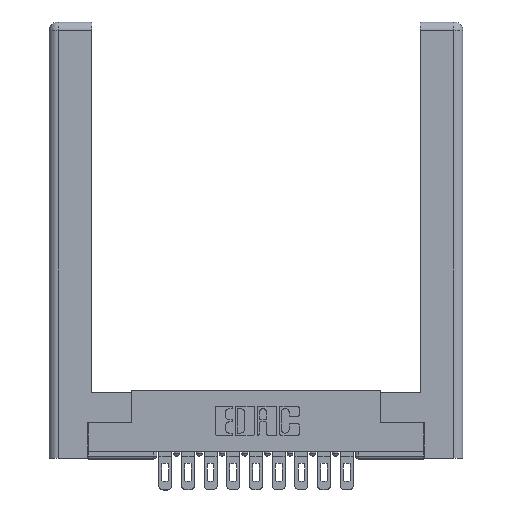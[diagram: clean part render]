
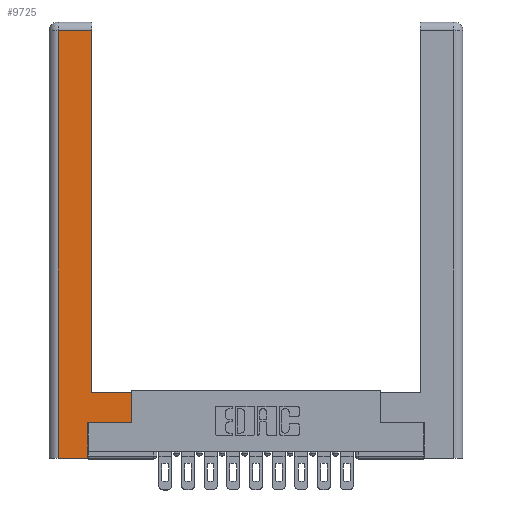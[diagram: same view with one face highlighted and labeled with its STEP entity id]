
A CAD part, top view. The second image highlights one B-rep face of the part: STEP entity #9725.
In plain terms, the highlighted planar face has unit normal (0, 0, 1).
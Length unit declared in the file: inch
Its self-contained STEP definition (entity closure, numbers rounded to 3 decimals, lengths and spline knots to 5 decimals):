
#487 = CARTESIAN_POINT ( 'NONE',  ( 0.0615, 2.94, 0. ) ) ;
#564 = LINE ( 'NONE', #487, #1114 ) ;
#850 = ORIENTED_EDGE ( 'NONE', *, *, #12295, .T. ) ;
#953 = ORIENTED_EDGE ( 'NONE', *, *, #1656, .T. ) ;
#957 = ORIENTED_EDGE ( 'NONE', *, *, #8066, .T. ) ;
#1100 = VERTEX_POINT ( 'NONE', #7253 ) ;
#1114 = VECTOR ( 'NONE', #5015, 39.37008 ) ;
#1339 = DIRECTION ( 'NONE',  ( 0., 0., -1. ) ) ;
#1393 = PLANE ( 'NONE',  #12175 ) ;
#1473 = LINE ( 'NONE', #10968, #13607 ) ;
#1656 = EDGE_CURVE ( 'NONE', #7311, #9506, #10340, .T. ) ;
#1848 = ORIENTED_EDGE ( 'NONE', *, *, #7405, .T. ) ;
#2497 = LINE ( 'NONE', #6456, #14647 ) ;
#2554 = CARTESIAN_POINT ( 'NONE',  ( 0., 0., 0. ) ) ;
#2973 = VECTOR ( 'NONE', #7549, 39.37008 ) ;
#3121 = EDGE_LOOP ( 'NONE', ( #14564, #850, #957, #953, #1848, #12884, #3713, #6019 ) ) ;
#3301 = VERTEX_POINT ( 'NONE', #11423 ) ;
#3435 = EDGE_CURVE ( 'NONE', #9109, #9801, #4992, .T. ) ;
#3713 = ORIENTED_EDGE ( 'NONE', *, *, #3435, .T. ) ;
#3739 = CARTESIAN_POINT ( 'NONE',  ( 0.0615, 0., 0. ) ) ;
#3912 = VECTOR ( 'NONE', #12351, 39.37008 ) ;
#4349 = CARTESIAN_POINT ( 'NONE',  ( 0.265, 0., 0. ) ) ;
#4493 = EDGE_CURVE ( 'NONE', #5567, #5960, #11987, .T. ) ;
#4613 = DIRECTION ( 'NONE',  ( 0., 1., 0. ) ) ;
#4992 = LINE ( 'NONE', #14107, #14067 ) ;
#5015 = DIRECTION ( 'NONE',  ( -1., 0., 0. ) ) ;
#5567 = VERTEX_POINT ( 'NONE', #13019 ) ;
#5960 = VERTEX_POINT ( 'NONE', #13094 ) ;
#6019 = ORIENTED_EDGE ( 'NONE', *, *, #14920, .T. ) ;
#6080 = CARTESIAN_POINT ( 'NONE',  ( 0.565, 0.245, 0. ) ) ;
#6351 = CARTESIAN_POINT ( 'NONE',  ( 0.565, 0.245, 0. ) ) ;
#6456 = CARTESIAN_POINT ( 'NONE',  ( 0.295, 0.45, 0. ) ) ;
#7253 = CARTESIAN_POINT ( 'NONE',  ( 0.265, 0.245, 0. ) ) ;
#7311 = VERTEX_POINT ( 'NONE', #3739 ) ;
#7330 = DIRECTION ( 'NONE',  ( 0., 1., 0. ) ) ;
#7405 = EDGE_CURVE ( 'NONE', #9506, #1100, #13794, .T. ) ;
#7549 = DIRECTION ( 'NONE',  ( 1., 0., 0. ) ) ;
#8066 = EDGE_CURVE ( 'NONE', #3301, #7311, #1473, .T. ) ;
#8740 = FACE_OUTER_BOUND ( 'NONE', #3121, .T. ) ;
#8805 = DIRECTION ( 'NONE',  ( 0., -1., 0. ) ) ;
#8833 = DIRECTION ( 'NONE',  ( -1., 0., 0. ) ) ;
#8848 = VECTOR ( 'NONE', #13304, 39.37008 ) ;
#9109 = VERTEX_POINT ( 'NONE', #6080 ) ;
#9506 = VERTEX_POINT ( 'NONE', #4349 ) ;
#9725 = ADVANCED_FACE ( 'NONE', ( #8740 ), #1393, .F. ) ;
#9801 = VERTEX_POINT ( 'NONE', #13140 ) ;
#10340 = LINE ( 'NONE', #12408, #2973 ) ;
#10623 = EDGE_CURVE ( 'NONE', #1100, #9109, #15177, .T. ) ;
#10968 = CARTESIAN_POINT ( 'NONE',  ( 0.0615, 0., 0. ) ) ;
#11423 = CARTESIAN_POINT ( 'NONE',  ( 0.0615, 2.94, 0. ) ) ;
#11957 = DIRECTION ( 'NONE',  ( -1., 0., 0. ) ) ;
#11987 = LINE ( 'NONE', #13399, #8848 ) ;
#12114 = VECTOR ( 'NONE', #7330, 39.37008 ) ;
#12175 = AXIS2_PLACEMENT_3D ( 'NONE', #2554, #1339, #11957 ) ;
#12295 = EDGE_CURVE ( 'NONE', #5960, #3301, #564, .T. ) ;
#12351 = DIRECTION ( 'NONE',  ( 1., 0., 0. ) ) ;
#12408 = CARTESIAN_POINT ( 'NONE',  ( 0.265, 0., 0. ) ) ;
#12884 = ORIENTED_EDGE ( 'NONE', *, *, #10623, .T. ) ;
#13019 = CARTESIAN_POINT ( 'NONE',  ( 0.295, 0.45, 0. ) ) ;
#13094 = CARTESIAN_POINT ( 'NONE',  ( 0.295, 2.94, 0. ) ) ;
#13140 = CARTESIAN_POINT ( 'NONE',  ( 0.565, 0.45, 0. ) ) ;
#13210 = CARTESIAN_POINT ( 'NONE',  ( 0.265, 0.245, 0. ) ) ;
#13304 = DIRECTION ( 'NONE',  ( 0., 1., 0. ) ) ;
#13399 = CARTESIAN_POINT ( 'NONE',  ( 0.295, 3., 0. ) ) ;
#13607 = VECTOR ( 'NONE', #8805, 39.37008 ) ;
#13794 = LINE ( 'NONE', #13210, #12114 ) ;
#14067 = VECTOR ( 'NONE', #4613, 39.37008 ) ;
#14107 = CARTESIAN_POINT ( 'NONE',  ( 0.565, 0.45, 0. ) ) ;
#14564 = ORIENTED_EDGE ( 'NONE', *, *, #4493, .T. ) ;
#14647 = VECTOR ( 'NONE', #8833, 39.37008 ) ;
#14920 = EDGE_CURVE ( 'NONE', #9801, #5567, #2497, .T. ) ;
#15177 = LINE ( 'NONE', #6351, #3912 ) ;
